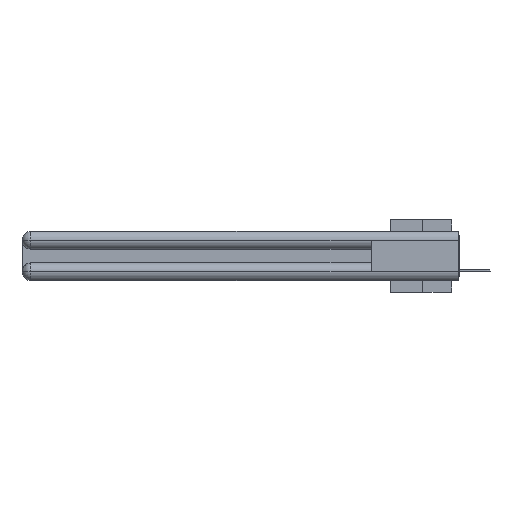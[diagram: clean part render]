
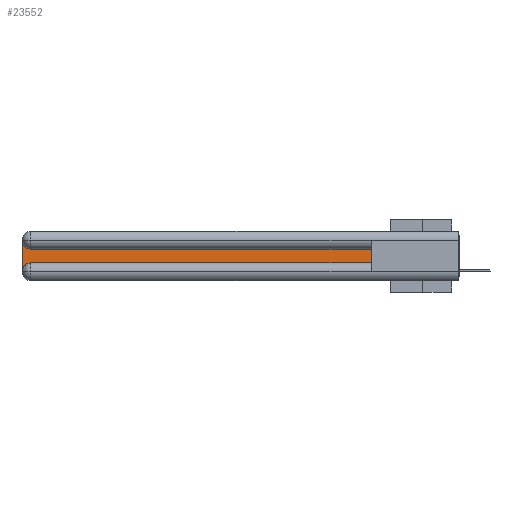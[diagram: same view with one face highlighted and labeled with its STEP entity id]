
A CAD part, left-side view. The second image highlights one B-rep face of the part: STEP entity #23552.
In plain terms, the highlighted planar face has unit normal (-1, 0, 0).
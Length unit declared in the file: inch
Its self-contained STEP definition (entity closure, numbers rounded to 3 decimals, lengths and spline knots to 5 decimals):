
#1510 = EDGE_CURVE ( 'NONE', #36031, #9901, #2124, .T. ) ;
#2124 = LINE ( 'NONE', #4733, #31483 ) ;
#2466 = CARTESIAN_POINT ( 'NONE',  ( 0.075, 2.94, -0.2775 ) ) ;
#2561 = ORIENTED_EDGE ( 'NONE', *, *, #33408, .T. ) ;
#3492 = EDGE_CURVE ( 'NONE', #9901, #8887, #26042, .T. ) ;
#3559 = DIRECTION ( 'NONE',  ( 0., 0., -1. ) ) ;
#3837 = EDGE_CURVE ( 'NONE', #17743, #16574, #32660, .T. ) ;
#4733 = CARTESIAN_POINT ( 'NONE',  ( 0.075, 3., -0.2175 ) ) ;
#5460 = DIRECTION ( 'NONE',  ( 0., 0., -1. ) ) ;
#6289 = VECTOR ( 'NONE', #11182, 39.37008 ) ;
#7965 = DIRECTION ( 'NONE',  ( 0., -1., 0. ) ) ;
#8024 = DIRECTION ( 'NONE',  ( 1., 0., 0. ) ) ;
#8855 = CARTESIAN_POINT ( 'NONE',  ( 0.075, 2.94, -0.1225 ) ) ;
#8887 = VERTEX_POINT ( 'NONE', #9894 ) ;
#9186 = LINE ( 'NONE', #13931, #35127 ) ;
#9894 = CARTESIAN_POINT ( 'NONE',  ( 0.075, 2.94, -0.2175 ) ) ;
#9901 = VERTEX_POINT ( 'NONE', #22865 ) ;
#10150 = ORIENTED_EDGE ( 'NONE', *, *, #28859, .T. ) ;
#11182 = DIRECTION ( 'NONE',  ( 0., 1., 0. ) ) ;
#11291 = CARTESIAN_POINT ( 'NONE',  ( 0.075, 0.6, -0.1225 ) ) ;
#13931 = CARTESIAN_POINT ( 'NONE',  ( 0.075, 0.6, -0.2175 ) ) ;
#15992 = VECTOR ( 'NONE', #7965, 39.37008 ) ;
#16027 = DIRECTION ( 'NONE',  ( 0., 0., -1. ) ) ;
#16574 = VERTEX_POINT ( 'NONE', #8855 ) ;
#16818 = CIRCLE ( 'NONE', #25660, 0.06 ) ;
#16873 = CARTESIAN_POINT ( 'NONE',  ( 0.075, 3., -0.1225 ) ) ;
#16990 = DIRECTION ( 'NONE',  ( 1., 0., 0. ) ) ;
#17350 = ORIENTED_EDGE ( 'NONE', *, *, #3837, .T. ) ;
#17743 = VERTEX_POINT ( 'NONE', #26640 ) ;
#20306 = EDGE_CURVE ( 'NONE', #8887, #21952, #26013, .T. ) ;
#20620 = DIRECTION ( 'NONE',  ( 1., 0., 0. ) ) ;
#20881 = ORIENTED_EDGE ( 'NONE', *, *, #1510, .T. ) ;
#21952 = VERTEX_POINT ( 'NONE', #22251 ) ;
#22251 = CARTESIAN_POINT ( 'NONE',  ( 0.075, 0.6, -0.2175 ) ) ;
#22675 = CARTESIAN_POINT ( 'NONE',  ( 0.075, 0.6, -0.2175 ) ) ;
#22865 = CARTESIAN_POINT ( 'NONE',  ( 0.075, 3., -0.2775 ) ) ;
#23458 = AXIS2_PLACEMENT_3D ( 'NONE', #2466, #8024, #33530 ) ;
#23552 = ADVANCED_FACE ( 'NONE', ( #36382 ), #25296, .F. ) ;
#24817 = ORIENTED_EDGE ( 'NONE', *, *, #3492, .T. ) ;
#25296 = PLANE ( 'NONE',  #28054 ) ;
#25660 = AXIS2_PLACEMENT_3D ( 'NONE', #26362, #20620, #3559 ) ;
#26013 = LINE ( 'NONE', #22675, #15992 ) ;
#26042 = CIRCLE ( 'NONE', #23458, 0.06 ) ;
#26362 = CARTESIAN_POINT ( 'NONE',  ( 0.075, 2.94, -0.0625 ) ) ;
#26640 = CARTESIAN_POINT ( 'NONE',  ( 0.075, 0.6, -0.1225 ) ) ;
#28054 = AXIS2_PLACEMENT_3D ( 'NONE', #16873, #16990, #5460 ) ;
#28859 = EDGE_CURVE ( 'NONE', #21952, #17743, #9186, .T. ) ;
#28946 = ORIENTED_EDGE ( 'NONE', *, *, #20306, .T. ) ;
#30681 = EDGE_LOOP ( 'NONE', ( #17350, #2561, #20881, #24817, #28946, #10150 ) ) ;
#31483 = VECTOR ( 'NONE', #16027, 39.37008 ) ;
#32660 = LINE ( 'NONE', #11291, #6289 ) ;
#33408 = EDGE_CURVE ( 'NONE', #16574, #36031, #16818, .T. ) ;
#33530 = DIRECTION ( 'NONE',  ( 0., 0., -1. ) ) ;
#33811 = CARTESIAN_POINT ( 'NONE',  ( 0.075, 3., -0.0625 ) ) ;
#33901 = DIRECTION ( 'NONE',  ( 0., 0., 1. ) ) ;
#35127 = VECTOR ( 'NONE', #33901, 39.37008 ) ;
#36031 = VERTEX_POINT ( 'NONE', #33811 ) ;
#36382 = FACE_OUTER_BOUND ( 'NONE', #30681, .T. ) ;
